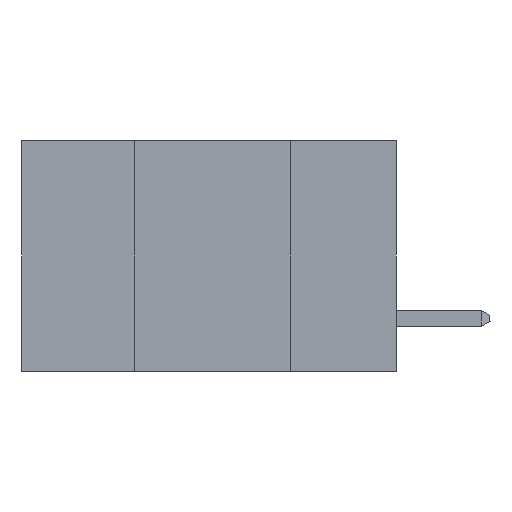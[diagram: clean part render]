
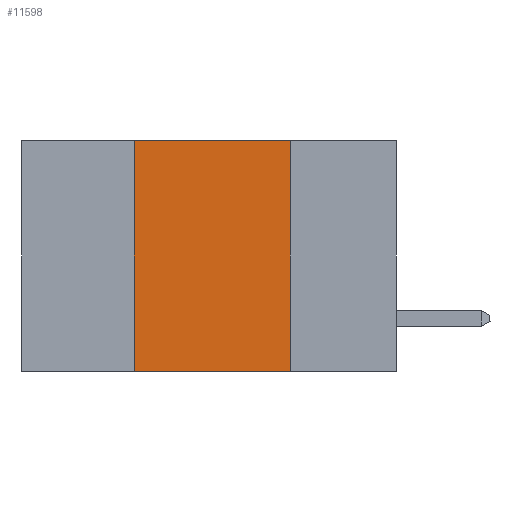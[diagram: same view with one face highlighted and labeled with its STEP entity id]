
A CAD part, left-side view. The second image highlights one B-rep face of the part: STEP entity #11598.
In plain terms, the highlighted planar face has unit normal (-1, 0, 0).
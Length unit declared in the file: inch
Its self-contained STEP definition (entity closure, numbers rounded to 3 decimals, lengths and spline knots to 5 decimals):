
#19 = CARTESIAN_POINT ( 'NONE',  ( 0., 0.42, 0. ) ) ;
#1123 = EDGE_LOOP ( 'NONE', ( #5279, #4968, #5928, #13628 ) ) ;
#1218 = DIRECTION ( 'NONE',  ( 0., 0., -1. ) ) ;
#1261 = LINE ( 'NONE', #22806, #5685 ) ;
#2264 = EDGE_CURVE ( 'NONE', #15994, #15536, #1261, .T. ) ;
#4683 = FACE_OUTER_BOUND ( 'NONE', #1123, .T. ) ;
#4800 = VERTEX_POINT ( 'NONE', #19 ) ;
#4956 = EDGE_CURVE ( 'NONE', #4800, #15994, #8465, .T. ) ;
#4968 = ORIENTED_EDGE ( 'NONE', *, *, #4956, .F. ) ;
#5279 = ORIENTED_EDGE ( 'NONE', *, *, #2264, .F. ) ;
#5389 = AXIS2_PLACEMENT_3D ( 'NONE', #7660, #9550, #22388 ) ;
#5685 = VECTOR ( 'NONE', #1218, 39.37008 ) ;
#5928 = ORIENTED_EDGE ( 'NONE', *, *, #23298, .F. ) ;
#6016 = CARTESIAN_POINT ( 'NONE',  ( 0., 0.42, -0.37 ) ) ;
#6192 = CARTESIAN_POINT ( 'NONE',  ( 0., 0.6, 0. ) ) ;
#7261 = CARTESIAN_POINT ( 'NONE',  ( 0., 0.42, 0. ) ) ;
#7660 = CARTESIAN_POINT ( 'NONE',  ( 0., 0.6, 0. ) ) ;
#8036 = DIRECTION ( 'NONE',  ( 0., -1., 0. ) ) ;
#8465 = LINE ( 'NONE', #6192, #22566 ) ;
#8615 = CARTESIAN_POINT ( 'NONE',  ( 0., 0.6, -0.37 ) ) ;
#9550 = DIRECTION ( 'NONE',  ( 1., 0., 0. ) ) ;
#9574 = VERTEX_POINT ( 'NONE', #6016 ) ;
#11598 = ADVANCED_FACE ( 'NONE', ( #4683 ), #20481, .F. ) ;
#12482 = VECTOR ( 'NONE', #23309, 39.37008 ) ;
#12590 = EDGE_CURVE ( 'NONE', #9574, #15536, #13047, .T. ) ;
#13047 = LINE ( 'NONE', #8615, #12482 ) ;
#13628 = ORIENTED_EDGE ( 'NONE', *, *, #12590, .T. ) ;
#14705 = VECTOR ( 'NONE', #18336, 39.37008 ) ;
#14814 = CARTESIAN_POINT ( 'NONE',  ( 0., 0.17, -0.37 ) ) ;
#15273 = LINE ( 'NONE', #7261, #14705 ) ;
#15536 = VERTEX_POINT ( 'NONE', #14814 ) ;
#15994 = VERTEX_POINT ( 'NONE', #18257 ) ;
#18257 = CARTESIAN_POINT ( 'NONE',  ( 0., 0.17, 0. ) ) ;
#18336 = DIRECTION ( 'NONE',  ( 0., 0., 1. ) ) ;
#20481 = PLANE ( 'NONE',  #5389 ) ;
#22388 = DIRECTION ( 'NONE',  ( 0., 0., -1. ) ) ;
#22566 = VECTOR ( 'NONE', #8036, 39.37008 ) ;
#22806 = CARTESIAN_POINT ( 'NONE',  ( 0., 0.17, 0. ) ) ;
#23298 = EDGE_CURVE ( 'NONE', #9574, #4800, #15273, .T. ) ;
#23309 = DIRECTION ( 'NONE',  ( 0., -1., 0. ) ) ;
